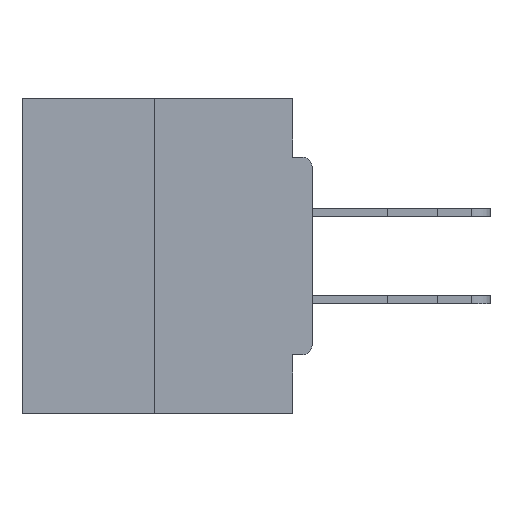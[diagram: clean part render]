
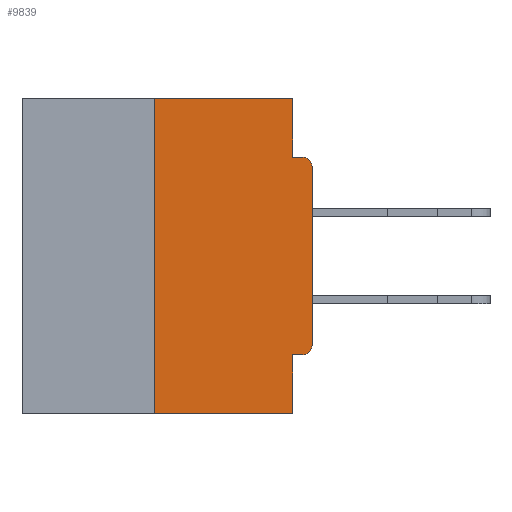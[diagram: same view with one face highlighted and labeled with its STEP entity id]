
A CAD part, left-side view. The second image highlights one B-rep face of the part: STEP entity #9839.
In plain terms, the highlighted planar face has unit normal (-1, 0, 0).
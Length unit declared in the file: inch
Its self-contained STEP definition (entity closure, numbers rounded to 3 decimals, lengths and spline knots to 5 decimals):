
#145 = EDGE_CURVE ( 'NONE', #365, #17118, #20613, .T. ) ;
#365 = VERTEX_POINT ( 'NONE', #5618 ) ;
#812 = VERTEX_POINT ( 'NONE', #34332 ) ;
#1898 = CARTESIAN_POINT ( 'NONE',  ( 0., 0.46, -0.5 ) ) ;
#2380 = PLANE ( 'NONE',  #5067 ) ;
#2453 = EDGE_CURVE ( 'NONE', #31537, #27132, #2529, .T. ) ;
#2459 = CARTESIAN_POINT ( 'NONE',  ( 0., 0.25, 0. ) ) ;
#2529 = LINE ( 'NONE', #13944, #19033 ) ;
#3187 = CARTESIAN_POINT ( 'NONE',  ( 0., 0., -0.1085 ) ) ;
#5051 = DIRECTION ( 'NONE',  ( 0., 0., -1. ) ) ;
#5067 = AXIS2_PLACEMENT_3D ( 'NONE', #25970, #14186, #17232 ) ;
#5618 = CARTESIAN_POINT ( 'NONE',  ( 0., 0.25, 0. ) ) ;
#5922 = LINE ( 'NONE', #2459, #18762 ) ;
#5973 = DIRECTION ( 'NONE',  ( 0., -1., 0. ) ) ;
#6237 = ORIENTED_EDGE ( 'NONE', *, *, #19575, .F. ) ;
#7170 = DIRECTION ( 'NONE',  ( 0., 1., 0. ) ) ;
#7334 = CARTESIAN_POINT ( 'NONE',  ( 0., 0.031, -0.4065 ) ) ;
#8051 = ORIENTED_EDGE ( 'NONE', *, *, #15870, .T. ) ;
#8659 = ORIENTED_EDGE ( 'NONE', *, *, #145, .F. ) ;
#9832 = EDGE_CURVE ( 'NONE', #17118, #11922, #35390, .T. ) ;
#9839 = ADVANCED_FACE ( 'NONE', ( #22996 ), #2380, .F. ) ;
#10624 = DIRECTION ( 'NONE',  ( -1., 0., 0. ) ) ;
#10857 = DIRECTION ( 'NONE',  ( 0., 0., 1. ) ) ;
#10880 = CIRCLE ( 'NONE', #16726, 0.015 ) ;
#11339 = VECTOR ( 'NONE', #7170, 39.37008 ) ;
#11922 = VERTEX_POINT ( 'NONE', #24881 ) ;
#13165 = CARTESIAN_POINT ( 'NONE',  ( 0., 0.031, 0. ) ) ;
#13210 = VECTOR ( 'NONE', #19361, 39.37008 ) ;
#13883 = LINE ( 'NONE', #31395, #23977 ) ;
#13944 = CARTESIAN_POINT ( 'NONE',  ( 0., 0., 0. ) ) ;
#14186 = DIRECTION ( 'NONE',  ( 1., 0., 0. ) ) ;
#15702 = EDGE_CURVE ( 'NONE', #23981, #22783, #22844, .T. ) ;
#15753 = EDGE_CURVE ( 'NONE', #11922, #812, #16844, .T. ) ;
#15870 = EDGE_CURVE ( 'NONE', #27132, #812, #10880, .T. ) ;
#16543 = VERTEX_POINT ( 'NONE', #7334 ) ;
#16719 = ORIENTED_EDGE ( 'NONE', *, *, #15753, .F. ) ;
#16726 = AXIS2_PLACEMENT_3D ( 'NONE', #27983, #10624, #31184 ) ;
#16844 = LINE ( 'NONE', #28643, #13210 ) ;
#16918 = VECTOR ( 'NONE', #28943, 39.37008 ) ;
#17118 = VERTEX_POINT ( 'NONE', #13165 ) ;
#17232 = DIRECTION ( 'NONE',  ( 0., 0., -1. ) ) ;
#18659 = EDGE_CURVE ( 'NONE', #23981, #365, #5922, .T. ) ;
#18759 = DIRECTION ( 'NONE',  ( -1., 0., 0. ) ) ;
#18762 = VECTOR ( 'NONE', #28670, 39.37008 ) ;
#19033 = VECTOR ( 'NONE', #10857, 39.37008 ) ;
#19140 = CARTESIAN_POINT ( 'NONE',  ( 0., 0.015, -0.3915 ) ) ;
#19361 = DIRECTION ( 'NONE',  ( 0., -1., 0. ) ) ;
#19575 = EDGE_CURVE ( 'NONE', #22465, #16543, #20985, .T. ) ;
#20016 = CARTESIAN_POINT ( 'NONE',  ( 0., 0.25, -0.5 ) ) ;
#20108 = EDGE_CURVE ( 'NONE', #22465, #31537, #22800, .T. ) ;
#20613 = LINE ( 'NONE', #25590, #16918 ) ;
#20985 = LINE ( 'NONE', #27876, #11339 ) ;
#21195 = CARTESIAN_POINT ( 'NONE',  ( 0., 0.015, -0.4065 ) ) ;
#22018 = EDGE_LOOP ( 'NONE', ( #8659, #31363, #26941, #34233, #6237, #23391, #28399, #8051, #16719, #36794 ) ) ;
#22465 = VERTEX_POINT ( 'NONE', #21195 ) ;
#22783 = VERTEX_POINT ( 'NONE', #28821 ) ;
#22800 = CIRCLE ( 'NONE', #34818, 0.015 ) ;
#22844 = LINE ( 'NONE', #1898, #37995 ) ;
#22996 = FACE_OUTER_BOUND ( 'NONE', #22018, .T. ) ;
#23391 = ORIENTED_EDGE ( 'NONE', *, *, #20108, .T. ) ;
#23977 = VECTOR ( 'NONE', #5051, 39.37008 ) ;
#23981 = VERTEX_POINT ( 'NONE', #20016 ) ;
#24881 = CARTESIAN_POINT ( 'NONE',  ( 0., 0.031, -0.0935 ) ) ;
#25590 = CARTESIAN_POINT ( 'NONE',  ( 0., 0.46, 0. ) ) ;
#25970 = CARTESIAN_POINT ( 'NONE',  ( 0., 0.46, 0. ) ) ;
#26941 = ORIENTED_EDGE ( 'NONE', *, *, #15702, .T. ) ;
#27132 = VERTEX_POINT ( 'NONE', #3187 ) ;
#27876 = CARTESIAN_POINT ( 'NONE',  ( 0., 0., -0.4065 ) ) ;
#27983 = CARTESIAN_POINT ( 'NONE',  ( 0., 0.015, -0.1085 ) ) ;
#28399 = ORIENTED_EDGE ( 'NONE', *, *, #2453, .T. ) ;
#28643 = CARTESIAN_POINT ( 'NONE',  ( 0., 0., -0.0935 ) ) ;
#28670 = DIRECTION ( 'NONE',  ( 0., 0., 1. ) ) ;
#28821 = CARTESIAN_POINT ( 'NONE',  ( 0., 0.031, -0.5 ) ) ;
#28848 = DIRECTION ( 'NONE',  ( 0., 0., -1. ) ) ;
#28943 = DIRECTION ( 'NONE',  ( 0., -1., 0. ) ) ;
#30840 = VECTOR ( 'NONE', #28848, 39.37008 ) ;
#30861 = EDGE_CURVE ( 'NONE', #16543, #22783, #13883, .T. ) ;
#31184 = DIRECTION ( 'NONE',  ( 0., 0., -1. ) ) ;
#31363 = ORIENTED_EDGE ( 'NONE', *, *, #18659, .F. ) ;
#31395 = CARTESIAN_POINT ( 'NONE',  ( 0., 0.031, -0.5 ) ) ;
#31536 = CARTESIAN_POINT ( 'NONE',  ( 0., 0.031, 0. ) ) ;
#31537 = VERTEX_POINT ( 'NONE', #34220 ) ;
#33568 = DIRECTION ( 'NONE',  ( 0., 0., -1. ) ) ;
#34220 = CARTESIAN_POINT ( 'NONE',  ( 0., 0., -0.3915 ) ) ;
#34233 = ORIENTED_EDGE ( 'NONE', *, *, #30861, .F. ) ;
#34332 = CARTESIAN_POINT ( 'NONE',  ( 0., 0.015, -0.0935 ) ) ;
#34818 = AXIS2_PLACEMENT_3D ( 'NONE', #19140, #18759, #33568 ) ;
#35390 = LINE ( 'NONE', #31536, #30840 ) ;
#36794 = ORIENTED_EDGE ( 'NONE', *, *, #9832, .F. ) ;
#37995 = VECTOR ( 'NONE', #5973, 39.37008 ) ;
